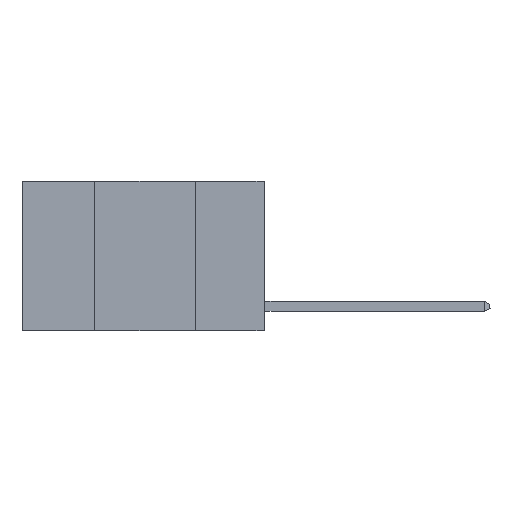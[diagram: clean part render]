
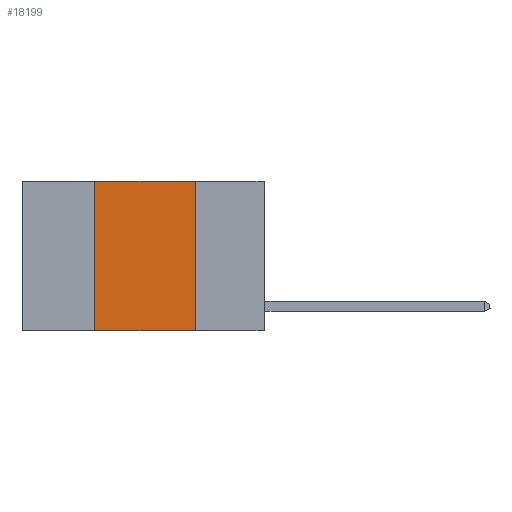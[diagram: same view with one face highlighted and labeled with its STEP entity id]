
A CAD part, left-side view. The second image highlights one B-rep face of the part: STEP entity #18199.
In plain terms, the highlighted planar face has unit normal (-1, 0, 0).
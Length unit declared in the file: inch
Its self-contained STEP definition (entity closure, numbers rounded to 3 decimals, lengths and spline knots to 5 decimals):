
#55 = VECTOR ( 'NONE', #13079, 39.37008 ) ;
#1100 = EDGE_LOOP ( 'NONE', ( #23737, #14095, #23225, #25977 ) ) ;
#1240 = DIRECTION ( 'NONE',  ( 0., -1., 0. ) ) ;
#1452 = LINE ( 'NONE', #1965, #17940 ) ;
#1965 = CARTESIAN_POINT ( 'NONE',  ( 0., 0.6, -0.37 ) ) ;
#2483 = CARTESIAN_POINT ( 'NONE',  ( 0., 0.42, 0. ) ) ;
#2697 = VERTEX_POINT ( 'NONE', #16759 ) ;
#3455 = CARTESIAN_POINT ( 'NONE',  ( 0., 0.6, 0. ) ) ;
#3570 = EDGE_CURVE ( 'NONE', #8169, #2697, #1452, .T. ) ;
#4174 = DIRECTION ( 'NONE',  ( 0., -1., 0. ) ) ;
#4328 = DIRECTION ( 'NONE',  ( 0., 0., -1. ) ) ;
#4366 = FACE_OUTER_BOUND ( 'NONE', #1100, .T. ) ;
#4426 = CARTESIAN_POINT ( 'NONE',  ( 0., 0.17, 0. ) ) ;
#4940 = LINE ( 'NONE', #2483, #15685 ) ;
#5136 = LINE ( 'NONE', #3455, #9532 ) ;
#8169 = VERTEX_POINT ( 'NONE', #9460 ) ;
#9413 = CARTESIAN_POINT ( 'NONE',  ( 0., 0.42, 0. ) ) ;
#9460 = CARTESIAN_POINT ( 'NONE',  ( 0., 0.42, -0.37 ) ) ;
#9532 = VECTOR ( 'NONE', #1240, 39.37008 ) ;
#10762 = EDGE_CURVE ( 'NONE', #26672, #17961, #5136, .T. ) ;
#11589 = LINE ( 'NONE', #4426, #55 ) ;
#11964 = DIRECTION ( 'NONE',  ( 0., 0., 1. ) ) ;
#12889 = CARTESIAN_POINT ( 'NONE',  ( 0., 0.6, 0. ) ) ;
#12958 = EDGE_CURVE ( 'NONE', #17961, #2697, #11589, .T. ) ;
#13079 = DIRECTION ( 'NONE',  ( 0., 0., -1. ) ) ;
#14095 = ORIENTED_EDGE ( 'NONE', *, *, #10762, .F. ) ;
#15024 = PLANE ( 'NONE',  #23540 ) ;
#15685 = VECTOR ( 'NONE', #11964, 39.37008 ) ;
#16759 = CARTESIAN_POINT ( 'NONE',  ( 0., 0.17, -0.37 ) ) ;
#17158 = DIRECTION ( 'NONE',  ( 1., 0., 0. ) ) ;
#17936 = EDGE_CURVE ( 'NONE', #8169, #26672, #4940, .T. ) ;
#17940 = VECTOR ( 'NONE', #4174, 39.37008 ) ;
#17961 = VERTEX_POINT ( 'NONE', #22649 ) ;
#18199 = ADVANCED_FACE ( 'NONE', ( #4366 ), #15024, .F. ) ;
#22649 = CARTESIAN_POINT ( 'NONE',  ( 0., 0.17, 0. ) ) ;
#23225 = ORIENTED_EDGE ( 'NONE', *, *, #17936, .F. ) ;
#23540 = AXIS2_PLACEMENT_3D ( 'NONE', #12889, #17158, #4328 ) ;
#23737 = ORIENTED_EDGE ( 'NONE', *, *, #12958, .F. ) ;
#25977 = ORIENTED_EDGE ( 'NONE', *, *, #3570, .T. ) ;
#26672 = VERTEX_POINT ( 'NONE', #9413 ) ;
